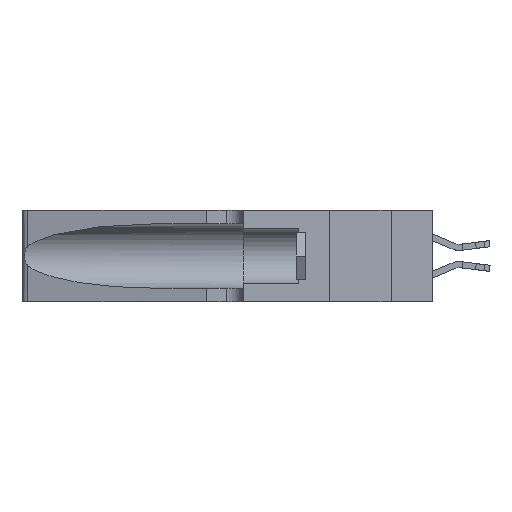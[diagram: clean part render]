
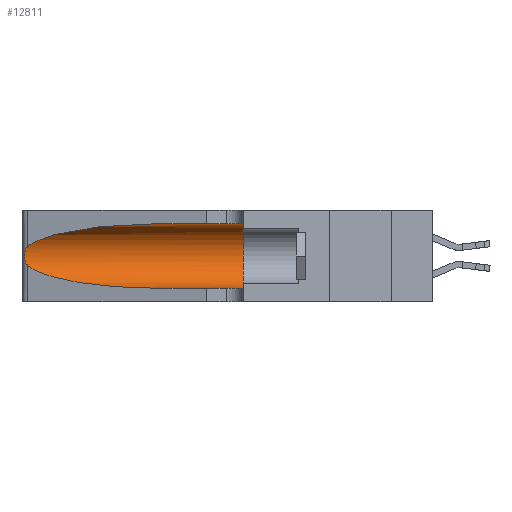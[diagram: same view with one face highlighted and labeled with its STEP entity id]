
A CAD part, left-side view. The second image highlights one B-rep face of the part: STEP entity #12811.
In plain terms, the highlighted cylindrical face has radius 3.308 mm (diameter 6.617 mm), a partial arc.
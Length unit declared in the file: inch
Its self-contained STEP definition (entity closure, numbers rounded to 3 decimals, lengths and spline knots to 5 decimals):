
#105 = CARTESIAN_POINT ( 'NONE',  ( 0.1305, 0.35, 0.185 ) ) ;
#217 = VECTOR ( 'NONE', #28357, 39.37008 ) ;
#837 = CYLINDRICAL_SURFACE ( 'NONE', #15996, 0.13025 ) ;
#935 = CARTESIAN_POINT ( 'NONE',  ( 0.25787, 1.23484, 0.2124 ) ) ;
#949 = LINE ( 'NONE', #14640, #217 ) ;
#1567 = CARTESIAN_POINT ( 'NONE',  ( 0.1305, 0.72297, 0.05475 ) ) ;
#2342 = CARTESIAN_POINT ( 'NONE',  ( 0.1305, 1.61858, 0.185 ) ) ;
#2459 = DIRECTION ( 'NONE',  ( 0., 0., 1. ) ) ;
#2861 = CARTESIAN_POINT ( 'NONE',  ( 0.2373, 1.15595, 0.28018 ) ) ;
#3332 = CARTESIAN_POINT ( 'NONE',  ( 0.26018, 1.23835, 0.19895 ) ) ;
#4359 = CARTESIAN_POINT ( 'NONE',  ( 0.1305, 0.72297, 0.31525 ) ) ;
#4361 = CARTESIAN_POINT ( 'NONE',  ( 0.2373, 1.15595, 0.08982 ) ) ;
#5109 = EDGE_CURVE ( 'NONE', #6990, #16077, #10166, .T. ) ;
#5644 = CARTESIAN_POINT ( 'NONE',  ( 0.26075, 1.23896, 0.178 ) ) ;
#6904 = VERTEX_POINT ( 'NONE', #17914 ) ;
#6948 = CARTESIAN_POINT ( 'NONE',  ( 0.1305, 0.35, 0.05475 ) ) ;
#6990 = VERTEX_POINT ( 'NONE', #25032 ) ;
#7937 = CARTESIAN_POINT ( 'NONE',  ( 0.25856, 1.23593, 0.16098 ) ) ;
#9200 = DIRECTION ( 'NONE',  ( 0., -1., 0. ) ) ;
#10151 = CARTESIAN_POINT ( 'NONE',  ( 0.25487, 1.22718, 0.22369 ) ) ;
#10166 =( BOUNDED_CURVE ( )  B_SPLINE_CURVE ( 3, ( #29561, #4361, #11158, #15877 ),
 .UNSPECIFIED., .F., .F. ) 
 B_SPLINE_CURVE_WITH_KNOTS ( ( 4, 4 ),
 ( 3.44316, 4.71239 ),
 .UNSPECIFIED. ) 
 CURVE ( )  GEOMETRIC_REPRESENTATION_ITEM ( )  RATIONAL_B_SPLINE_CURVE ( ( 1., 0.87, 0.87, 1. ) ) 
 REPRESENTATION_ITEM ( '' )  );
#10255 = CARTESIAN_POINT ( 'NONE',  ( 0.25639, 1.23186, 0.15144 ) ) ;
#10935 = DIRECTION ( 'NONE',  ( 0., -1., 0. ) ) ;
#11158 = CARTESIAN_POINT ( 'NONE',  ( 0.18966, 0.96281, 0.05475 ) ) ;
#12555 = CARTESIAN_POINT ( 'NONE',  ( 0.25487, 1.22718, 0.14631 ) ) ;
#12708 = AXIS2_PLACEMENT_3D ( 'NONE', #105, #16243, #2459 ) ;
#12811 = ADVANCED_FACE ( 'NONE', ( #13132 ), #837, .F. ) ;
#13132 = FACE_OUTER_BOUND ( 'NONE', #19460, .T. ) ;
#13375 = ORIENTED_EDGE ( 'NONE', *, *, #26573, .T. ) ;
#13643 = CIRCLE ( 'NONE', #12708, 0.13025 ) ;
#13668 = ORIENTED_EDGE ( 'NONE', *, *, #18849, .F. ) ;
#13934 = ORIENTED_EDGE ( 'NONE', *, *, #26962, .F. ) ;
#14309 = CARTESIAN_POINT ( 'NONE',  ( 0.18966, 0.96281, 0.31525 ) ) ;
#14640 = CARTESIAN_POINT ( 'NONE',  ( 0.1305, 1.61858, 0.05475 ) ) ;
#14761 = CARTESIAN_POINT ( 'NONE',  ( 0.25639, 1.23184, 0.21858 ) ) ;
#15485 = VERTEX_POINT ( 'NONE', #4359 ) ;
#15665 = VERTEX_POINT ( 'NONE', #27786 ) ;
#15877 = CARTESIAN_POINT ( 'NONE',  ( 0.1305, 0.72297, 0.05475 ) ) ;
#15996 = AXIS2_PLACEMENT_3D ( 'NONE', #2342, #9200, #18418 ) ;
#16077 = VERTEX_POINT ( 'NONE', #1567 ) ;
#16243 = DIRECTION ( 'NONE',  ( 0., 1., 0. ) ) ;
#16429 = EDGE_CURVE ( 'NONE', #15485, #15665, #23216, .T. ) ;
#17069 = CARTESIAN_POINT ( 'NONE',  ( 0.25854, 1.2359, 0.20912 ) ) ;
#17914 = CARTESIAN_POINT ( 'NONE',  ( 0.1305, 0.35, 0.31525 ) ) ;
#18418 = DIRECTION ( 'NONE',  ( 0., 0., -1. ) ) ;
#18649 = VECTOR ( 'NONE', #10935, 39.37008 ) ;
#18849 = EDGE_CURVE ( 'NONE', #15485, #6904, #24074, .T. ) ;
#18916 = CARTESIAN_POINT ( 'NONE',  ( 0.25487, 1.22718, 0.22369 ) ) ;
#19354 = CARTESIAN_POINT ( 'NONE',  ( 0.26075, 1.23896, 0.19203 ) ) ;
#19460 = EDGE_LOOP ( 'NONE', ( #25617, #13375, #28219, #28969, #13934, #13668 ) ) ;
#20130 = VERTEX_POINT ( 'NONE', #6948 ) ;
#20395 = EDGE_CURVE ( 'NONE', #16077, #20130, #949, .T. ) ;
#20896 = B_SPLINE_CURVE_WITH_KNOTS ( 'NONE', 3,
 ( #10151, #23918, #14761, #935, #17069, #3332, #19354, #5644, #21678, #7937, #24013, #10255, #26316, #12555 ),
 .UNSPECIFIED., .F., .F.,
 ( 4, 2, 2, 2, 2, 2, 4 ),
 ( 0., 0.00027, 0.00053, 0.00107, 0.0016, 0.00187, 0.00214 ),
 .UNSPECIFIED. ) ;
#21678 = CARTESIAN_POINT ( 'NONE',  ( 0.26017, 1.23833, 0.17102 ) ) ;
#22375 = CARTESIAN_POINT ( 'NONE',  ( 0.1305, 1.61858, 0.31525 ) ) ;
#23216 =( BOUNDED_CURVE ( )  B_SPLINE_CURVE ( 3, ( #25773, #14309, #2861, #18916 ),
 .UNSPECIFIED., .F., .T. ) 
 B_SPLINE_CURVE_WITH_KNOTS ( ( 4, 4 ),
 ( 1.5708, 2.84003 ),
 .UNSPECIFIED. ) 
 CURVE ( )  GEOMETRIC_REPRESENTATION_ITEM ( )  RATIONAL_B_SPLINE_CURVE ( ( 1., 0.87, 0.87, 1. ) ) 
 REPRESENTATION_ITEM ( '' )  );
#23918 = CARTESIAN_POINT ( 'NONE',  ( 0.25555, 1.22994, 0.2215 ) ) ;
#24013 = CARTESIAN_POINT ( 'NONE',  ( 0.25789, 1.23486, 0.15765 ) ) ;
#24074 = LINE ( 'NONE', #22375, #18649 ) ;
#25032 = CARTESIAN_POINT ( 'NONE',  ( 0.25487, 1.22718, 0.14631 ) ) ;
#25617 = ORIENTED_EDGE ( 'NONE', *, *, #16429, .T. ) ;
#25773 = CARTESIAN_POINT ( 'NONE',  ( 0.1305, 0.72297, 0.31525 ) ) ;
#26316 = CARTESIAN_POINT ( 'NONE',  ( 0.25555, 1.22993, 0.14849 ) ) ;
#26573 = EDGE_CURVE ( 'NONE', #15665, #6990, #20896, .T. ) ;
#26962 = EDGE_CURVE ( 'NONE', #6904, #20130, #13643, .T. ) ;
#27786 = CARTESIAN_POINT ( 'NONE',  ( 0.25487, 1.22718, 0.22369 ) ) ;
#28219 = ORIENTED_EDGE ( 'NONE', *, *, #5109, .T. ) ;
#28357 = DIRECTION ( 'NONE',  ( 0., -1., 0. ) ) ;
#28969 = ORIENTED_EDGE ( 'NONE', *, *, #20395, .T. ) ;
#29561 = CARTESIAN_POINT ( 'NONE',  ( 0.25487, 1.22718, 0.14631 ) ) ;
